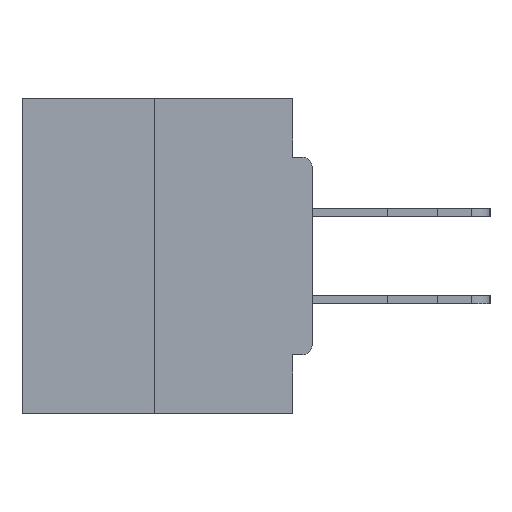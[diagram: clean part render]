
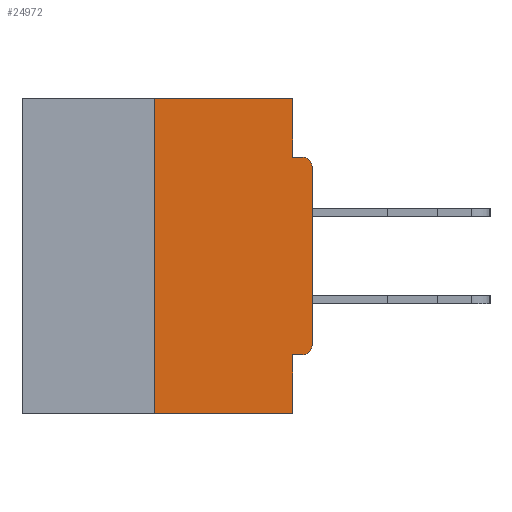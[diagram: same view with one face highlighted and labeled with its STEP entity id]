
A CAD part, left-side view. The second image highlights one B-rep face of the part: STEP entity #24972.
In plain terms, the highlighted planar face has unit normal (-1, 0, 0).
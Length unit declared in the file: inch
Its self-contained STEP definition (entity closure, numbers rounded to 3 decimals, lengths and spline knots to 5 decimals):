
#348 = ORIENTED_EDGE ( 'NONE', *, *, #13367, .F. ) ;
#545 = CARTESIAN_POINT ( 'NONE',  ( 0., 0.46, -0.5 ) ) ;
#552 = CARTESIAN_POINT ( 'NONE',  ( 0., 0.031, -0.5 ) ) ;
#1044 = LINE ( 'NONE', #8960, #9949 ) ;
#1074 = CARTESIAN_POINT ( 'NONE',  ( 0., 0.015, -0.0935 ) ) ;
#1936 = DIRECTION ( 'NONE',  ( 0., 0., -1. ) ) ;
#2699 = ORIENTED_EDGE ( 'NONE', *, *, #15643, .F. ) ;
#2729 = ORIENTED_EDGE ( 'NONE', *, *, #8819, .F. ) ;
#3128 = CARTESIAN_POINT ( 'NONE',  ( 0., 0.25, 0. ) ) ;
#3482 = DIRECTION ( 'NONE',  ( 0., 0., 1. ) ) ;
#3553 = VERTEX_POINT ( 'NONE', #28130 ) ;
#3849 = EDGE_CURVE ( 'NONE', #34103, #27131, #19518, .T. ) ;
#4304 = VECTOR ( 'NONE', #3482, 39.37008 ) ;
#4354 = ORIENTED_EDGE ( 'NONE', *, *, #33300, .T. ) ;
#4602 = DIRECTION ( 'NONE',  ( 0., 0., -1. ) ) ;
#4779 = CARTESIAN_POINT ( 'NONE',  ( 0., 0.015, -0.1085 ) ) ;
#5022 = DIRECTION ( 'NONE',  ( 0., 1., 0. ) ) ;
#6006 = VECTOR ( 'NONE', #32925, 39.37008 ) ;
#6106 = ORIENTED_EDGE ( 'NONE', *, *, #3849, .T. ) ;
#6387 = ORIENTED_EDGE ( 'NONE', *, *, #32162, .F. ) ;
#6929 = DIRECTION ( 'NONE',  ( -1., 0., 0. ) ) ;
#7305 = VERTEX_POINT ( 'NONE', #10717 ) ;
#7516 = VERTEX_POINT ( 'NONE', #25559 ) ;
#7657 = ORIENTED_EDGE ( 'NONE', *, *, #7675, .T. ) ;
#7659 = EDGE_CURVE ( 'NONE', #7305, #25068, #19608, .T. ) ;
#7675 = EDGE_CURVE ( 'NONE', #27131, #7305, #12459, .T. ) ;
#7904 = AXIS2_PLACEMENT_3D ( 'NONE', #14527, #30801, #30977 ) ;
#7935 = VERTEX_POINT ( 'NONE', #33548 ) ;
#8413 = LINE ( 'NONE', #19147, #34858 ) ;
#8794 = LINE ( 'NONE', #545, #6006 ) ;
#8819 = EDGE_CURVE ( 'NONE', #3553, #22234, #33112, .T. ) ;
#8960 = CARTESIAN_POINT ( 'NONE',  ( 0., 0., -0.0935 ) ) ;
#9468 = VECTOR ( 'NONE', #10012, 39.37008 ) ;
#9949 = VECTOR ( 'NONE', #19880, 39.37008 ) ;
#10012 = DIRECTION ( 'NONE',  ( 0., -1., 0. ) ) ;
#10717 = CARTESIAN_POINT ( 'NONE',  ( 0., 0., -0.1085 ) ) ;
#11007 = AXIS2_PLACEMENT_3D ( 'NONE', #4779, #6929, #4602 ) ;
#11130 = PLANE ( 'NONE',  #7904 ) ;
#11310 = FACE_OUTER_BOUND ( 'NONE', #28519, .T. ) ;
#12459 = LINE ( 'NONE', #29289, #13304 ) ;
#13031 = CARTESIAN_POINT ( 'NONE',  ( 0., 0.031, 0. ) ) ;
#13304 = VECTOR ( 'NONE', #23227, 39.37008 ) ;
#13367 = EDGE_CURVE ( 'NONE', #34103, #3553, #8413, .T. ) ;
#13580 = CARTESIAN_POINT ( 'NONE',  ( 0., 0.015, -0.3915 ) ) ;
#13763 = DIRECTION ( 'NONE',  ( 0., 0., -1. ) ) ;
#13783 = CARTESIAN_POINT ( 'NONE',  ( 0., 0.031, 0. ) ) ;
#14527 = CARTESIAN_POINT ( 'NONE',  ( 0., 0.46, 0. ) ) ;
#15576 = CARTESIAN_POINT ( 'NONE',  ( 0., 0.46, 0. ) ) ;
#15643 = EDGE_CURVE ( 'NONE', #7516, #7935, #19790, .T. ) ;
#17132 = DIRECTION ( 'NONE',  ( -1., 0., 0. ) ) ;
#18878 = EDGE_CURVE ( 'NONE', #23084, #29034, #28975, .T. ) ;
#19104 = CARTESIAN_POINT ( 'NONE',  ( 0., 0., -0.3915 ) ) ;
#19147 = CARTESIAN_POINT ( 'NONE',  ( 0., 0., -0.4065 ) ) ;
#19518 = CIRCLE ( 'NONE', #21220, 0.015 ) ;
#19608 = CIRCLE ( 'NONE', #11007, 0.015 ) ;
#19790 = LINE ( 'NONE', #3128, #4304 ) ;
#19880 = DIRECTION ( 'NONE',  ( 0., -1., 0. ) ) ;
#20228 = CARTESIAN_POINT ( 'NONE',  ( 0., 0.015, -0.4065 ) ) ;
#20847 = ORIENTED_EDGE ( 'NONE', *, *, #7659, .T. ) ;
#21220 = AXIS2_PLACEMENT_3D ( 'NONE', #13580, #17132, #13763 ) ;
#22234 = VERTEX_POINT ( 'NONE', #27346 ) ;
#22414 = DIRECTION ( 'NONE',  ( 0., 0., -1. ) ) ;
#23084 = VERTEX_POINT ( 'NONE', #13783 ) ;
#23227 = DIRECTION ( 'NONE',  ( 0., 0., 1. ) ) ;
#24972 = ADVANCED_FACE ( 'NONE', ( #11310 ), #11130, .F. ) ;
#25068 = VERTEX_POINT ( 'NONE', #1074 ) ;
#25559 = CARTESIAN_POINT ( 'NONE',  ( 0., 0.25, -0.5 ) ) ;
#27131 = VERTEX_POINT ( 'NONE', #19104 ) ;
#27346 = CARTESIAN_POINT ( 'NONE',  ( 0., 0.031, -0.5 ) ) ;
#28130 = CARTESIAN_POINT ( 'NONE',  ( 0., 0.031, -0.4065 ) ) ;
#28213 = CARTESIAN_POINT ( 'NONE',  ( 0., 0.031, -0.0935 ) ) ;
#28519 = EDGE_LOOP ( 'NONE', ( #29907, #2699, #4354, #2729, #348, #6106, #7657, #20847, #6387, #31683 ) ) ;
#28975 = LINE ( 'NONE', #13031, #29385 ) ;
#29034 = VERTEX_POINT ( 'NONE', #28213 ) ;
#29289 = CARTESIAN_POINT ( 'NONE',  ( 0., 0., 0. ) ) ;
#29385 = VECTOR ( 'NONE', #1936, 39.37008 ) ;
#29907 = ORIENTED_EDGE ( 'NONE', *, *, #34305, .F. ) ;
#30145 = VECTOR ( 'NONE', #22414, 39.37008 ) ;
#30801 = DIRECTION ( 'NONE',  ( 1., 0., 0. ) ) ;
#30977 = DIRECTION ( 'NONE',  ( 0., 0., -1. ) ) ;
#31683 = ORIENTED_EDGE ( 'NONE', *, *, #18878, .F. ) ;
#32162 = EDGE_CURVE ( 'NONE', #29034, #25068, #1044, .T. ) ;
#32925 = DIRECTION ( 'NONE',  ( 0., -1., 0. ) ) ;
#33112 = LINE ( 'NONE', #552, #30145 ) ;
#33300 = EDGE_CURVE ( 'NONE', #7516, #22234, #8794, .T. ) ;
#33548 = CARTESIAN_POINT ( 'NONE',  ( 0., 0.25, 0. ) ) ;
#34103 = VERTEX_POINT ( 'NONE', #20228 ) ;
#34305 = EDGE_CURVE ( 'NONE', #7935, #23084, #34690, .T. ) ;
#34690 = LINE ( 'NONE', #15576, #9468 ) ;
#34858 = VECTOR ( 'NONE', #5022, 39.37008 ) ;
